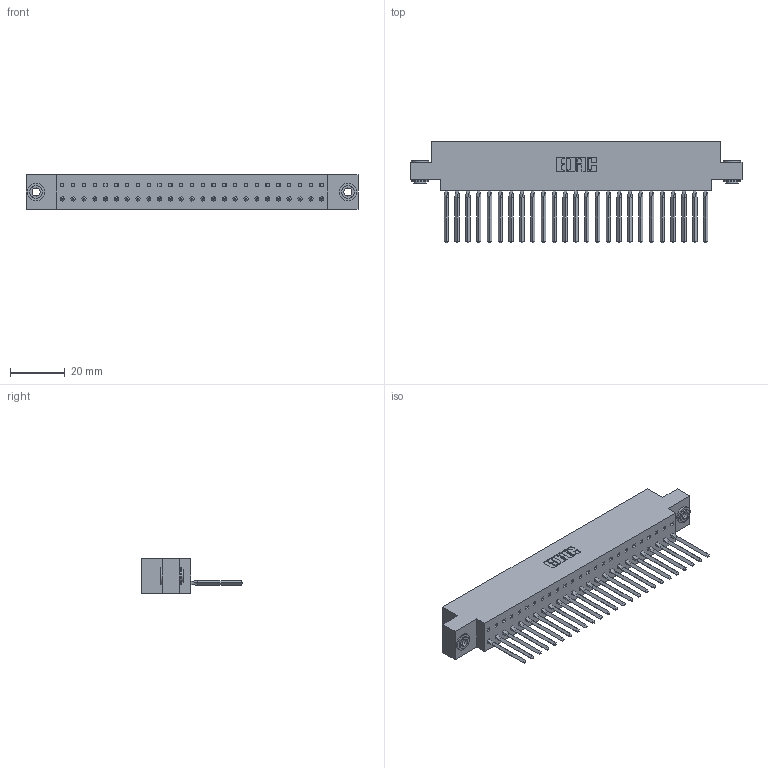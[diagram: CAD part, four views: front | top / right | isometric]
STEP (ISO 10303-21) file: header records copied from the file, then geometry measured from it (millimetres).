
FILE_DESCRIPTION (( 'STEP AP203' ), '1' );
FILE_NAME ('317-025-541-603.STEP', '2020-02-27T18:29:35', ( '' ), ( '' ), 'SwSTEP 2.0', 'SolidWorks 2016', '' );
FILE_SCHEMA (( 'CONFIG_CONTROL_DESIGN' ));
Length unit declared in the file: inch
Products named in the file (4): 317 Part_.156 Dia - TH; 345-250-002_345-250-002-102; 317-025-541-603; 317-290-002_541
Assembly tree (28 placements, depth 2):
  317-025-541-603
    317 Part_.156 Dia - TH
    317-290-002_541  x25
    345-250-002_345-250-002-102  x2
Bounding box: 121.77 x 37.34 x 12.7 mm (x, y, z)
Volume: 19243.3 mm3; surface area: 26840 mm2
Topology: 28 solids, 28 shells, 3940 faces, 11201 edges, 7280 vertices
Faces by surface type: plane 3168, cylinder 664, bspline 100, cone 8
Entity records: 39907 total; most frequent: CARTESIAN_POINT 7695, ORIENTED_EDGE 6966, DIRECTION 5751, EDGE_CURVE 3483, LINE 3095, VECTOR 3095, VERTEX_POINT 2312, AXIS2_PLACEMENT_3D 1328
